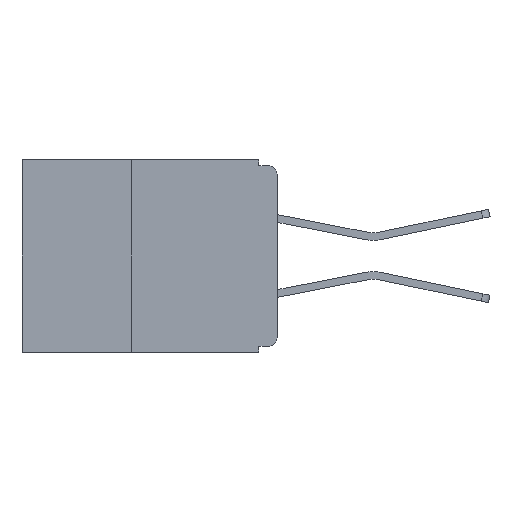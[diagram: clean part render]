
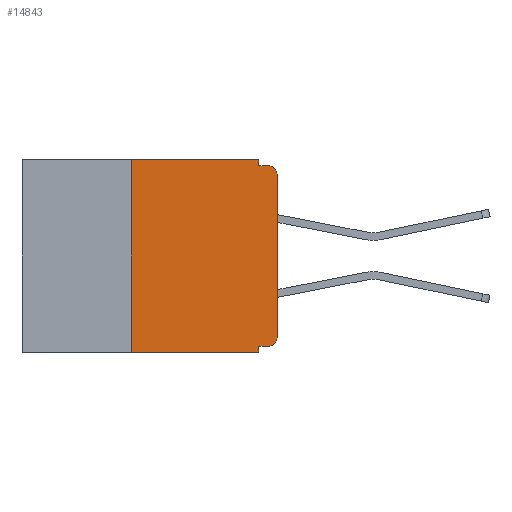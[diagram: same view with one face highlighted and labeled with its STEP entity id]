
A CAD part, left-side view. The second image highlights one B-rep face of the part: STEP entity #14843.
In plain terms, the highlighted planar face has unit normal (-1, 0, 0).
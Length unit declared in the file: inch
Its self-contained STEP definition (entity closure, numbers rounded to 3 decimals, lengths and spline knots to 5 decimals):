
#695 = CARTESIAN_POINT ( 'NONE',  ( 0., 0.25, 0. ) ) ;
#712 = FACE_OUTER_BOUND ( 'NONE', #9569, .T. ) ;
#920 = DIRECTION ( 'NONE',  ( 0., 0., -1. ) ) ;
#1046 = CARTESIAN_POINT ( 'NONE',  ( 0., 0.25, -0.33 ) ) ;
#1290 = DIRECTION ( 'NONE',  ( 0., 0., -1. ) ) ;
#1616 = EDGE_CURVE ( 'NONE', #6707, #9359, #21509, .T. ) ;
#1702 = CARTESIAN_POINT ( 'NONE',  ( 0., 0., -0.32 ) ) ;
#2967 = VECTOR ( 'NONE', #920, 39.37008 ) ;
#3378 = ORIENTED_EDGE ( 'NONE', *, *, #14714, .F. ) ;
#3509 = AXIS2_PLACEMENT_3D ( 'NONE', #5111, #5053, #6160 ) ;
#3546 = CARTESIAN_POINT ( 'NONE',  ( 0., 0., -0.305 ) ) ;
#3815 = LINE ( 'NONE', #7949, #22147 ) ;
#3963 = ORIENTED_EDGE ( 'NONE', *, *, #13526, .F. ) ;
#4669 = CARTESIAN_POINT ( 'NONE',  ( 0., 0.031, 0. ) ) ;
#5053 = DIRECTION ( 'NONE',  ( -1., 0., 0. ) ) ;
#5111 = CARTESIAN_POINT ( 'NONE',  ( 0., 0.015, -0.305 ) ) ;
#5230 = EDGE_CURVE ( 'NONE', #15273, #14860, #7882, .T. ) ;
#5331 = ORIENTED_EDGE ( 'NONE', *, *, #20723, .T. ) ;
#6160 = DIRECTION ( 'NONE',  ( 0., 0., -1. ) ) ;
#6183 = ORIENTED_EDGE ( 'NONE', *, *, #7661, .F. ) ;
#6633 = PLANE ( 'NONE',  #8210 ) ;
#6707 = VERTEX_POINT ( 'NONE', #9822 ) ;
#7114 = CARTESIAN_POINT ( 'NONE',  ( 0., 0.031, -0.01 ) ) ;
#7661 = EDGE_CURVE ( 'NONE', #6707, #23082, #17800, .T. ) ;
#7752 = LINE ( 'NONE', #13449, #2967 ) ;
#7882 = CIRCLE ( 'NONE', #18892, 0.015 ) ;
#7949 = CARTESIAN_POINT ( 'NONE',  ( 0., 0., 0. ) ) ;
#8066 = VERTEX_POINT ( 'NONE', #4669 ) ;
#8210 = AXIS2_PLACEMENT_3D ( 'NONE', #8429, #12109, #1290 ) ;
#8429 = CARTESIAN_POINT ( 'NONE',  ( 0., 0.437, 0. ) ) ;
#8475 = CARTESIAN_POINT ( 'NONE',  ( 0., 0.031, -0.33 ) ) ;
#8502 = CARTESIAN_POINT ( 'NONE',  ( 0., 0.015, -0.01 ) ) ;
#8566 = LINE ( 'NONE', #19208, #12856 ) ;
#8904 = DIRECTION ( 'NONE',  ( 0., 1., 0. ) ) ;
#9262 = ORIENTED_EDGE ( 'NONE', *, *, #12327, .T. ) ;
#9280 = VECTOR ( 'NONE', #20906, 39.37008 ) ;
#9359 = VERTEX_POINT ( 'NONE', #3546 ) ;
#9569 = EDGE_LOOP ( 'NONE', ( #5331, #20088, #12405, #3378, #12977, #3963, #9262, #19248, #6183, #12704 ) ) ;
#9812 = DIRECTION ( 'NONE',  ( 0., 0., 1. ) ) ;
#9822 = CARTESIAN_POINT ( 'NONE',  ( 0., 0.015, -0.32 ) ) ;
#10209 = VERTEX_POINT ( 'NONE', #695 ) ;
#10428 = CARTESIAN_POINT ( 'NONE',  ( 0., 0., -0.025 ) ) ;
#11125 = EDGE_CURVE ( 'NONE', #23082, #17204, #13551, .T. ) ;
#11220 = VECTOR ( 'NONE', #12319, 39.37008 ) ;
#11982 = CARTESIAN_POINT ( 'NONE',  ( 0., 0.437, -0.33 ) ) ;
#12109 = DIRECTION ( 'NONE',  ( 1., 0., 0. ) ) ;
#12319 = DIRECTION ( 'NONE',  ( 0., -1., 0. ) ) ;
#12327 = EDGE_CURVE ( 'NONE', #22197, #17204, #16748, .T. ) ;
#12405 = ORIENTED_EDGE ( 'NONE', *, *, #13703, .F. ) ;
#12704 = ORIENTED_EDGE ( 'NONE', *, *, #1616, .T. ) ;
#12856 = VECTOR ( 'NONE', #22735, 39.37008 ) ;
#12977 = ORIENTED_EDGE ( 'NONE', *, *, #20276, .F. ) ;
#13449 = CARTESIAN_POINT ( 'NONE',  ( 0., 0.031, 0. ) ) ;
#13526 = EDGE_CURVE ( 'NONE', #22197, #10209, #15119, .T. ) ;
#13551 = LINE ( 'NONE', #8475, #9280 ) ;
#13703 = EDGE_CURVE ( 'NONE', #19755, #14860, #20563, .T. ) ;
#14581 = VECTOR ( 'NONE', #15406, 39.37008 ) ;
#14714 = EDGE_CURVE ( 'NONE', #8066, #19755, #7752, .T. ) ;
#14763 = DIRECTION ( 'NONE',  ( 0., 0., -1. ) ) ;
#14805 = DIRECTION ( 'NONE',  ( -1., 0., 0. ) ) ;
#14809 = CARTESIAN_POINT ( 'NONE',  ( 0., 0.015, -0.025 ) ) ;
#14843 = ADVANCED_FACE ( 'NONE', ( #712 ), #6633, .F. ) ;
#14860 = VERTEX_POINT ( 'NONE', #8502 ) ;
#15119 = LINE ( 'NONE', #1046, #14581 ) ;
#15166 = CARTESIAN_POINT ( 'NONE',  ( 0., 0.031, -0.32 ) ) ;
#15273 = VERTEX_POINT ( 'NONE', #10428 ) ;
#15406 = DIRECTION ( 'NONE',  ( 0., 0., 1. ) ) ;
#15772 = CARTESIAN_POINT ( 'NONE',  ( 0., 0., -0.01 ) ) ;
#16179 = CARTESIAN_POINT ( 'NONE',  ( 0., 0.25, -0.33 ) ) ;
#16748 = LINE ( 'NONE', #11982, #22513 ) ;
#17204 = VERTEX_POINT ( 'NONE', #21325 ) ;
#17238 = VECTOR ( 'NONE', #8904, 39.37008 ) ;
#17800 = LINE ( 'NONE', #1702, #17238 ) ;
#18892 = AXIS2_PLACEMENT_3D ( 'NONE', #14809, #14805, #14763 ) ;
#19208 = CARTESIAN_POINT ( 'NONE',  ( 0., 0.437, 0. ) ) ;
#19248 = ORIENTED_EDGE ( 'NONE', *, *, #11125, .F. ) ;
#19755 = VERTEX_POINT ( 'NONE', #7114 ) ;
#20088 = ORIENTED_EDGE ( 'NONE', *, *, #5230, .T. ) ;
#20276 = EDGE_CURVE ( 'NONE', #10209, #8066, #8566, .T. ) ;
#20563 = LINE ( 'NONE', #15772, #11220 ) ;
#20723 = EDGE_CURVE ( 'NONE', #9359, #15273, #3815, .T. ) ;
#20906 = DIRECTION ( 'NONE',  ( 0., 0., -1. ) ) ;
#21325 = CARTESIAN_POINT ( 'NONE',  ( 0., 0.031, -0.33 ) ) ;
#21509 = CIRCLE ( 'NONE', #3509, 0.015 ) ;
#22147 = VECTOR ( 'NONE', #9812, 39.37008 ) ;
#22197 = VERTEX_POINT ( 'NONE', #16179 ) ;
#22402 = DIRECTION ( 'NONE',  ( 0., -1., 0. ) ) ;
#22513 = VECTOR ( 'NONE', #22402, 39.37008 ) ;
#22735 = DIRECTION ( 'NONE',  ( 0., -1., 0. ) ) ;
#23082 = VERTEX_POINT ( 'NONE', #15166 ) ;
